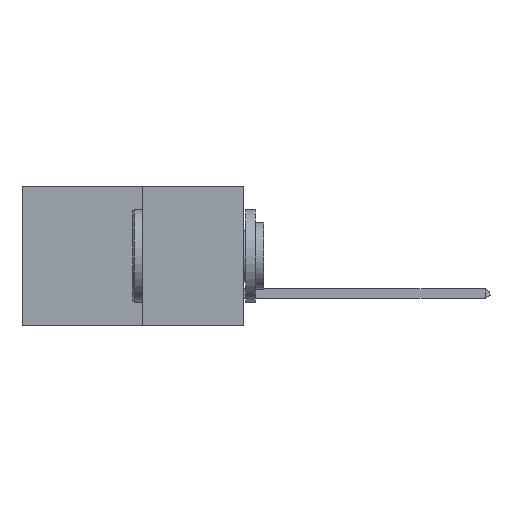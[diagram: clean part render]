
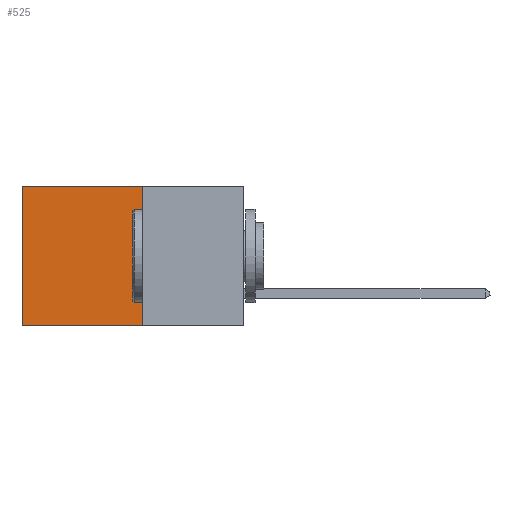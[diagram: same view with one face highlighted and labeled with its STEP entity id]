
A CAD part, left-side view. The second image highlights one B-rep face of the part: STEP entity #525.
In plain terms, the highlighted planar face has unit normal (-1, 0, 0).
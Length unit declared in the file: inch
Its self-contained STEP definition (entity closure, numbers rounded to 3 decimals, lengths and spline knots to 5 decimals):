
#40 = VECTOR ( 'NONE', #21161, 39.37008 ) ;
#525 = ADVANCED_FACE ( 'NONE', ( #7375 ), #5958, .F. ) ;
#561 = DIRECTION ( 'NONE',  ( 0., 1., 0. ) ) ;
#2033 = VERTEX_POINT ( 'NONE', #21831 ) ;
#2293 = AXIS2_PLACEMENT_3D ( 'NONE', #12823, #9756, #5866 ) ;
#2374 = VERTEX_POINT ( 'NONE', #17986 ) ;
#3970 = CARTESIAN_POINT ( 'NONE',  ( 0.277, 0.59, -0.37 ) ) ;
#5866 = DIRECTION ( 'NONE',  ( 0., 0., -1. ) ) ;
#5958 = PLANE ( 'NONE',  #2293 ) ;
#6619 = CARTESIAN_POINT ( 'NONE',  ( 0.277, 0.27, -0.37 ) ) ;
#7375 = FACE_OUTER_BOUND ( 'NONE', #13115, .T. ) ;
#8672 = EDGE_CURVE ( 'NONE', #2033, #2374, #22167, .T. ) ;
#9535 = VERTEX_POINT ( 'NONE', #6619 ) ;
#9756 = DIRECTION ( 'NONE',  ( 1., 0., 0. ) ) ;
#10899 = LINE ( 'NONE', #17858, #19499 ) ;
#11506 = ORIENTED_EDGE ( 'NONE', *, *, #20525, .F. ) ;
#11610 = CARTESIAN_POINT ( 'NONE',  ( 0.277, 0.27, 0. ) ) ;
#11758 = CARTESIAN_POINT ( 'NONE',  ( 0.277, 0.59, -0.37 ) ) ;
#12507 = EDGE_CURVE ( 'NONE', #9535, #15643, #10899, .T. ) ;
#12823 = CARTESIAN_POINT ( 'NONE',  ( 0.277, 0.27, -0.37 ) ) ;
#13115 = EDGE_LOOP ( 'NONE', ( #21250, #17604, #11506, #22172 ) ) ;
#13568 = VECTOR ( 'NONE', #15141, 39.37008 ) ;
#13875 = LINE ( 'NONE', #3970, #40 ) ;
#15141 = DIRECTION ( 'NONE',  ( 0., 1., 0. ) ) ;
#15300 = DIRECTION ( 'NONE',  ( 0., 0., -1. ) ) ;
#15305 = EDGE_CURVE ( 'NONE', #2374, #15643, #13875, .T. ) ;
#15643 = VERTEX_POINT ( 'NONE', #11758 ) ;
#16073 = VECTOR ( 'NONE', #15300, 39.37008 ) ;
#16620 = LINE ( 'NONE', #17054, #16073 ) ;
#17054 = CARTESIAN_POINT ( 'NONE',  ( 0.277, 0.27, -0.37 ) ) ;
#17604 = ORIENTED_EDGE ( 'NONE', *, *, #12507, .F. ) ;
#17858 = CARTESIAN_POINT ( 'NONE',  ( 0.277, 0.27, -0.37 ) ) ;
#17986 = CARTESIAN_POINT ( 'NONE',  ( 0.277, 0.59, 0. ) ) ;
#19499 = VECTOR ( 'NONE', #561, 39.37008 ) ;
#20525 = EDGE_CURVE ( 'NONE', #2033, #9535, #16620, .T. ) ;
#21161 = DIRECTION ( 'NONE',  ( 0., 0., -1. ) ) ;
#21250 = ORIENTED_EDGE ( 'NONE', *, *, #15305, .T. ) ;
#21831 = CARTESIAN_POINT ( 'NONE',  ( 0.277, 0.27, 0. ) ) ;
#22167 = LINE ( 'NONE', #11610, #13568 ) ;
#22172 = ORIENTED_EDGE ( 'NONE', *, *, #8672, .T. ) ;
